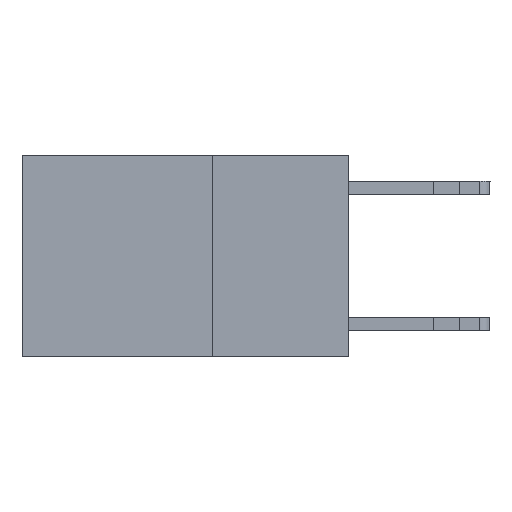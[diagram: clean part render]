
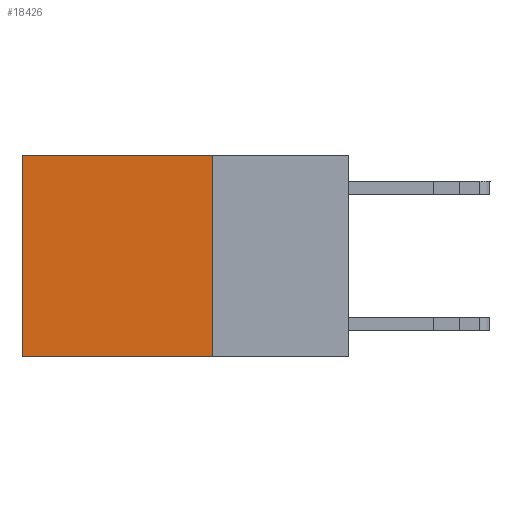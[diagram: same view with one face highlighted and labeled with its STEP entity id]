
A CAD part, left-side view. The second image highlights one B-rep face of the part: STEP entity #18426.
In plain terms, the highlighted planar face has unit normal (-1, 0, 0).
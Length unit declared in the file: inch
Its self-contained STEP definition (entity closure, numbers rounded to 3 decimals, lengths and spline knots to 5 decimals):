
#30 = LINE ( 'NONE', #14239, #17713 ) ;
#320 = CARTESIAN_POINT ( 'NONE',  ( 0.2625, 0.6, -0.37 ) ) ;
#346 = PLANE ( 'NONE',  #4480 ) ;
#449 = DIRECTION ( 'NONE',  ( 0., 0., -1. ) ) ;
#549 = CARTESIAN_POINT ( 'NONE',  ( 0.2625, 0.6, 0. ) ) ;
#1126 = VERTEX_POINT ( 'NONE', #5810 ) ;
#1195 = VECTOR ( 'NONE', #4548, 39.37008 ) ;
#1749 = VERTEX_POINT ( 'NONE', #2499 ) ;
#2499 = CARTESIAN_POINT ( 'NONE',  ( 0.2625, 0.25, -0.37 ) ) ;
#2601 = VERTEX_POINT ( 'NONE', #6471 ) ;
#4415 = ORIENTED_EDGE ( 'NONE', *, *, #7801, .T. ) ;
#4480 = AXIS2_PLACEMENT_3D ( 'NONE', #14558, #13239, #449 ) ;
#4548 = DIRECTION ( 'NONE',  ( 0., 1., 0. ) ) ;
#4981 = EDGE_CURVE ( 'NONE', #1749, #10079, #12875, .T. ) ;
#5072 = EDGE_CURVE ( 'NONE', #1126, #2601, #11568, .T. ) ;
#5810 = CARTESIAN_POINT ( 'NONE',  ( 0.2625, 0.25, 0. ) ) ;
#5943 = CARTESIAN_POINT ( 'NONE',  ( 0.2625, 0.25, 0. ) ) ;
#5988 = DIRECTION ( 'NONE',  ( 0., 0., -1. ) ) ;
#6267 = EDGE_LOOP ( 'NONE', ( #4415, #12665, #14006, #12638 ) ) ;
#6471 = CARTESIAN_POINT ( 'NONE',  ( 0.2625, 0.6, 0. ) ) ;
#6860 = VECTOR ( 'NONE', #12791, 39.37008 ) ;
#7517 = VECTOR ( 'NONE', #7793, 39.37008 ) ;
#7793 = DIRECTION ( 'NONE',  ( 0., 0., -1. ) ) ;
#7801 = EDGE_CURVE ( 'NONE', #2601, #10079, #9123, .T. ) ;
#8470 = CARTESIAN_POINT ( 'NONE',  ( 0.2625, 0.25, -0.37 ) ) ;
#9123 = LINE ( 'NONE', #549, #7517 ) ;
#10079 = VERTEX_POINT ( 'NONE', #320 ) ;
#11568 = LINE ( 'NONE', #5943, #1195 ) ;
#11639 = FACE_OUTER_BOUND ( 'NONE', #6267, .T. ) ;
#12472 = EDGE_CURVE ( 'NONE', #1126, #1749, #30, .T. ) ;
#12638 = ORIENTED_EDGE ( 'NONE', *, *, #5072, .T. ) ;
#12665 = ORIENTED_EDGE ( 'NONE', *, *, #4981, .F. ) ;
#12791 = DIRECTION ( 'NONE',  ( 0., 1., 0. ) ) ;
#12875 = LINE ( 'NONE', #8470, #6860 ) ;
#13239 = DIRECTION ( 'NONE',  ( 1., 0., 0. ) ) ;
#14006 = ORIENTED_EDGE ( 'NONE', *, *, #12472, .F. ) ;
#14239 = CARTESIAN_POINT ( 'NONE',  ( 0.2625, 0.25, 0. ) ) ;
#14558 = CARTESIAN_POINT ( 'NONE',  ( 0.2625, 0.25, 0. ) ) ;
#17713 = VECTOR ( 'NONE', #5988, 39.37008 ) ;
#18426 = ADVANCED_FACE ( 'NONE', ( #11639 ), #346, .F. ) ;
